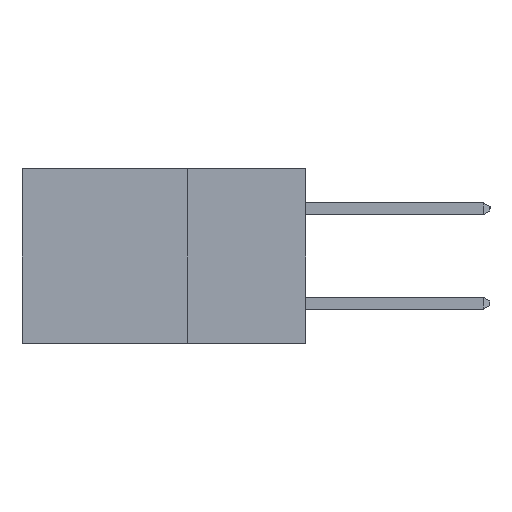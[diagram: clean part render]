
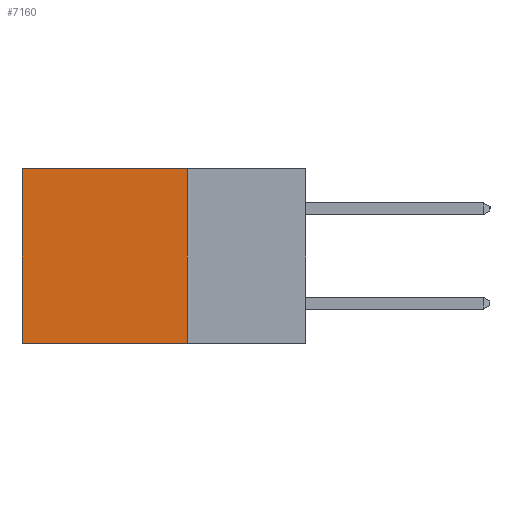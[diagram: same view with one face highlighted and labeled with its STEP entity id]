
A CAD part, left-side view. The second image highlights one B-rep face of the part: STEP entity #7160.
In plain terms, the highlighted planar face has unit normal (-1, 0, 0).
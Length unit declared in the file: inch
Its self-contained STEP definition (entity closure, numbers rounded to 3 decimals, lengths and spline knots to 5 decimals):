
#109 = DIRECTION ( 'NONE',  ( 0., 0., -1. ) ) ;
#1016 = LINE ( 'NONE', #6879, #8844 ) ;
#1278 = CARTESIAN_POINT ( 'NONE',  ( 0.2615, 0.25, -0.37 ) ) ;
#1515 = VECTOR ( 'NONE', #109, 39.37008 ) ;
#1518 = DIRECTION ( 'NONE',  ( 0., 0., -1. ) ) ;
#1724 = AXIS2_PLACEMENT_3D ( 'NONE', #9578, #7321, #1518 ) ;
#2025 = VERTEX_POINT ( 'NONE', #8456 ) ;
#2436 = LINE ( 'NONE', #1278, #1515 ) ;
#3135 = VERTEX_POINT ( 'NONE', #12676 ) ;
#3295 = VECTOR ( 'NONE', #3336, 39.37008 ) ;
#3336 = DIRECTION ( 'NONE',  ( 0., 1., 0. ) ) ;
#3830 = PLANE ( 'NONE',  #1724 ) ;
#5076 = EDGE_CURVE ( 'NONE', #2025, #3135, #1016, .T. ) ;
#5276 = CARTESIAN_POINT ( 'NONE',  ( 0.2615, 0.25, 0. ) ) ;
#5661 = VERTEX_POINT ( 'NONE', #14722 ) ;
#5754 = EDGE_LOOP ( 'NONE', ( #7702, #6523, #6693, #6841 ) ) ;
#6523 = ORIENTED_EDGE ( 'NONE', *, *, #11150, .F. ) ;
#6693 = ORIENTED_EDGE ( 'NONE', *, *, #8814, .F. ) ;
#6841 = ORIENTED_EDGE ( 'NONE', *, *, #14967, .T. ) ;
#6879 = CARTESIAN_POINT ( 'NONE',  ( 0.2615, 0.6, -0.37 ) ) ;
#7160 = ADVANCED_FACE ( 'NONE', ( #14561 ), #3830, .F. ) ;
#7308 = CARTESIAN_POINT ( 'NONE',  ( 0.2615, 0.25, 0. ) ) ;
#7321 = DIRECTION ( 'NONE',  ( 1., 0., 0. ) ) ;
#7702 = ORIENTED_EDGE ( 'NONE', *, *, #5076, .T. ) ;
#8456 = CARTESIAN_POINT ( 'NONE',  ( 0.2615, 0.6, 0. ) ) ;
#8814 = EDGE_CURVE ( 'NONE', #14101, #5661, #2436, .T. ) ;
#8844 = VECTOR ( 'NONE', #15137, 39.37008 ) ;
#9073 = LINE ( 'NONE', #13748, #3295 ) ;
#9516 = VECTOR ( 'NONE', #9704, 39.37008 ) ;
#9578 = CARTESIAN_POINT ( 'NONE',  ( 0.2615, 0.25, -0.37 ) ) ;
#9704 = DIRECTION ( 'NONE',  ( 0., 1., 0. ) ) ;
#11150 = EDGE_CURVE ( 'NONE', #5661, #3135, #9073, .T. ) ;
#12676 = CARTESIAN_POINT ( 'NONE',  ( 0.2615, 0.6, -0.37 ) ) ;
#13070 = LINE ( 'NONE', #7308, #9516 ) ;
#13748 = CARTESIAN_POINT ( 'NONE',  ( 0.2615, 0.25, -0.37 ) ) ;
#14101 = VERTEX_POINT ( 'NONE', #5276 ) ;
#14561 = FACE_OUTER_BOUND ( 'NONE', #5754, .T. ) ;
#14722 = CARTESIAN_POINT ( 'NONE',  ( 0.2615, 0.25, -0.37 ) ) ;
#14967 = EDGE_CURVE ( 'NONE', #14101, #2025, #13070, .T. ) ;
#15137 = DIRECTION ( 'NONE',  ( 0., 0., -1. ) ) ;
